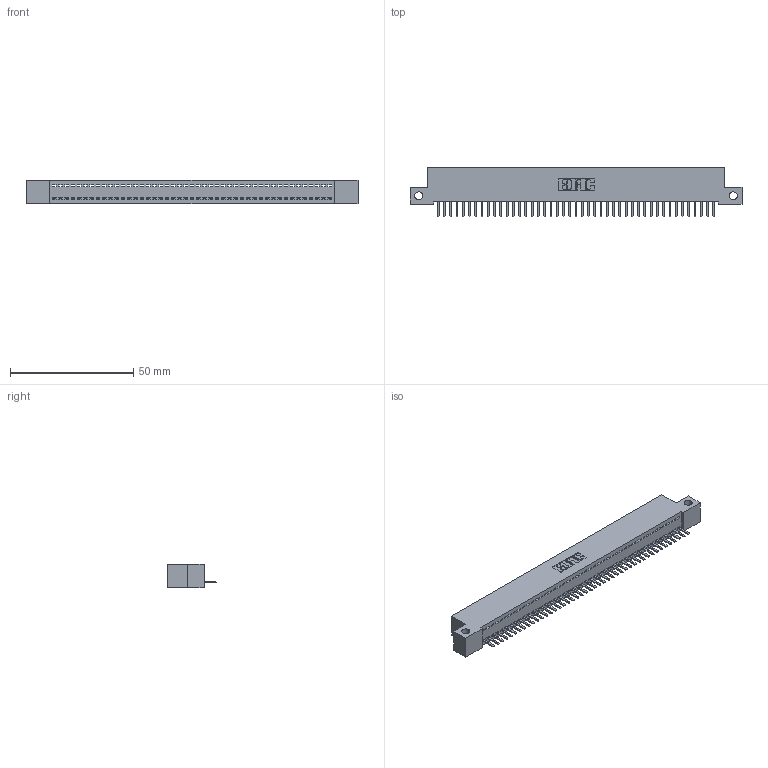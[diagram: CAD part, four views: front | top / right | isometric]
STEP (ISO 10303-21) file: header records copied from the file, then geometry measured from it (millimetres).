
FILE_DESCRIPTION (( 'STEP AP203' ), '1' );
FILE_NAME ('392-045-520-112.STEP', '2018-08-16T15:51:35', ( '' ), ( '' ), 'SwSTEP 2.0', 'SolidWorks 2016', '' );
FILE_SCHEMA (( 'CONFIG_CONTROL_DESIGN' ));
Length unit declared in the file: inch
Products named in the file (3): 392-045-520-112; 342 Part_Side Mount; 345-292-001_345-293-120
Assembly tree (46 placements, depth 2):
  392-045-520-112
    342 Part_Side Mount
    345-292-001_345-293-120  x45
Bounding box: 134.62 x 20.02 x 9.4 mm (x, y, z)
Volume: 11611.2 mm3; surface area: 16529.4 mm2
Topology: 46 solids, 46 shells, 2900 faces, 8579 edges, 5598 vertices
Faces by surface type: plane 2046, cylinder 854
Entity records: 27107 total; most frequent: CARTESIAN_POINT 4693, ORIENTED_EDGE 4662, DIRECTION 3941, EDGE_CURVE 2331, LINE 2199, VECTOR 2199, VERTEX_POINT 1550, AXIS2_PLACEMENT_3D 871
